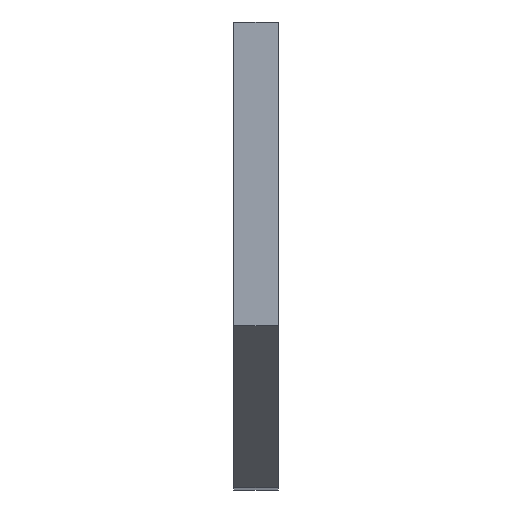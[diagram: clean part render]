
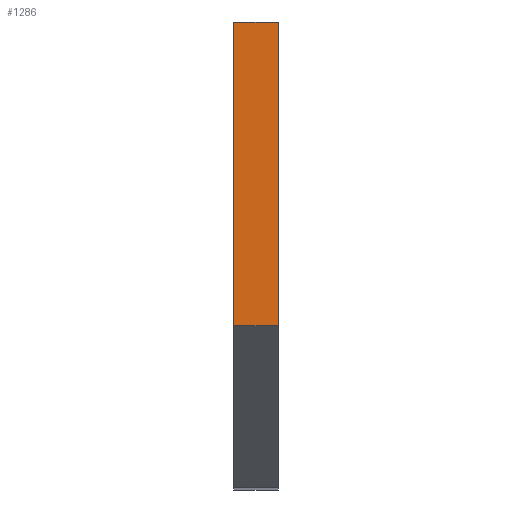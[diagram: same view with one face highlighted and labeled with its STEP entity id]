
A CAD part, top view. The second image highlights one B-rep face of the part: STEP entity #1286.
In plain terms, the highlighted planar face has unit normal (0, 0, 1).
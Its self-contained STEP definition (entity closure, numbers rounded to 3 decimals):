
#9 = VERTEX_POINT ( 'NONE', #187 ) ;
#84 = ORIENTED_EDGE ( 'NONE', *, *, #1169, .F. ) ;
#146 = CARTESIAN_POINT ( 'NONE',  ( 0., 33.426, 0. ) ) ;
#180 = DIRECTION ( 'NONE',  ( 0., 0., -1. ) ) ;
#187 = CARTESIAN_POINT ( 'NONE',  ( 0., 11.608, 0. ) ) ;
#203 = DIRECTION ( 'NONE',  ( 0., -1., 0. ) ) ;
#246 = FACE_OUTER_BOUND ( 'NONE', #847, .T. ) ;
#252 = CARTESIAN_POINT ( 'NONE',  ( 3.175, 11.608, 0. ) ) ;
#277 = PLANE ( 'NONE',  #768 ) ;
#284 = CARTESIAN_POINT ( 'NONE',  ( 3.175, 33.426, 0. ) ) ;
#291 = EDGE_CURVE ( 'NONE', #1307, #331, #311, .T. ) ;
#311 = LINE ( 'NONE', #769, #1365 ) ;
#331 = VERTEX_POINT ( 'NONE', #146 ) ;
#337 = ORIENTED_EDGE ( 'NONE', *, *, #1006, .T. ) ;
#367 = VERTEX_POINT ( 'NONE', #252 ) ;
#465 = DIRECTION ( 'NONE',  ( -1., 0., 0. ) ) ;
#533 = CARTESIAN_POINT ( 'NONE',  ( 3.175, 0., 0. ) ) ;
#549 = DIRECTION ( 'NONE',  ( -1., 0., 0. ) ) ;
#565 = LINE ( 'NONE', #722, #1123 ) ;
#587 = CARTESIAN_POINT ( 'NONE',  ( 3.175, 0., 0. ) ) ;
#603 = ORIENTED_EDGE ( 'NONE', *, *, #765, .F. ) ;
#616 = LINE ( 'NONE', #533, #1109 ) ;
#722 = CARTESIAN_POINT ( 'NONE',  ( 0., 0., 0. ) ) ;
#735 = LINE ( 'NONE', #1186, #1007 ) ;
#762 = ORIENTED_EDGE ( 'NONE', *, *, #291, .T. ) ;
#765 = EDGE_CURVE ( 'NONE', #367, #9, #735, .T. ) ;
#768 = AXIS2_PLACEMENT_3D ( 'NONE', #587, #180, #898 ) ;
#769 = CARTESIAN_POINT ( 'NONE',  ( 3.175, 33.426, 0. ) ) ;
#847 = EDGE_LOOP ( 'NONE', ( #337, #603, #84, #762 ) ) ;
#898 = DIRECTION ( 'NONE',  ( 0., 1., 0. ) ) ;
#952 = DIRECTION ( 'NONE',  ( 0., -1., 0. ) ) ;
#1006 = EDGE_CURVE ( 'NONE', #331, #9, #565, .T. ) ;
#1007 = VECTOR ( 'NONE', #465, 1000. ) ;
#1109 = VECTOR ( 'NONE', #952, 1000. ) ;
#1123 = VECTOR ( 'NONE', #203, 1000. ) ;
#1169 = EDGE_CURVE ( 'NONE', #1307, #367, #616, .T. ) ;
#1186 = CARTESIAN_POINT ( 'NONE',  ( 3.175, 11.608, 0. ) ) ;
#1286 = ADVANCED_FACE ( 'NONE', ( #246 ), #277, .F. ) ;
#1307 = VERTEX_POINT ( 'NONE', #284 ) ;
#1365 = VECTOR ( 'NONE', #549, 1000. ) ;
